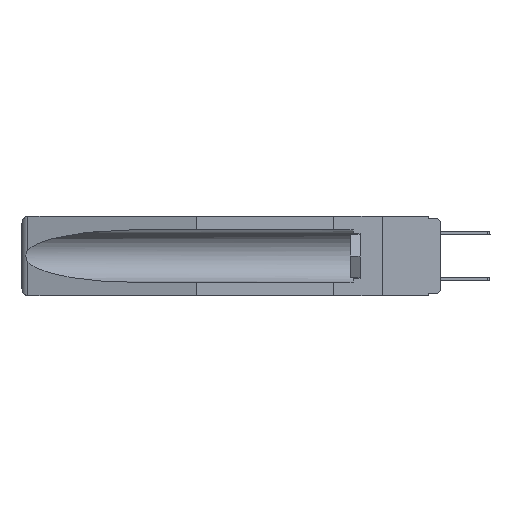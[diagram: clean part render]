
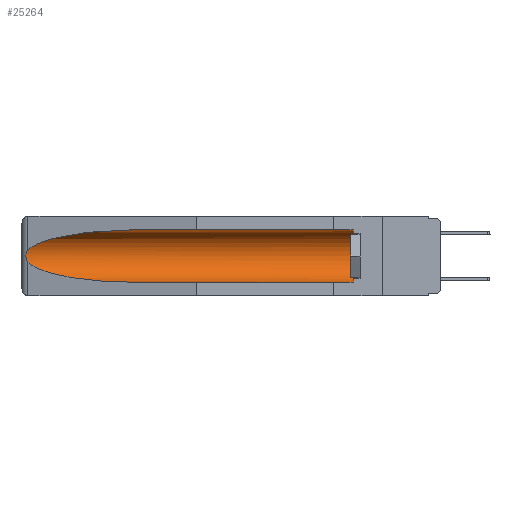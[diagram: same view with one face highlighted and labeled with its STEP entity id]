
A CAD part, left-side view. The second image highlights one B-rep face of the part: STEP entity #25264.
In plain terms, the highlighted cylindrical face has radius 2.857 mm (diameter 5.715 mm), a partial arc.
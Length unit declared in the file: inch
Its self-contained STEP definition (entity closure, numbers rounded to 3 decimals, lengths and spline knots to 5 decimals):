
#78 = CARTESIAN_POINT ( 'NONE',  ( 0.155, 0.126, -0.284 ) ) ;
#177 = DIRECTION ( 'NONE',  ( 0., 0., 1. ) ) ;
#429 = ORIENTED_EDGE ( 'NONE', *, *, #6052, .T. ) ;
#585 = EDGE_CURVE ( 'NONE', #12339, #21316, #16014, .T. ) ;
#729 = LINE ( 'NONE', #15188, #16115 ) ;
#1210 = CARTESIAN_POINT ( 'NONE',  ( 0.155, 1.07973, -0.059 ) ) ;
#1318 = CARTESIAN_POINT ( 'NONE',  ( 0.21114, 1.30732, -0.059 ) ) ;
#1515 = CARTESIAN_POINT ( 'NONE',  ( 0.25451, 1.48313, -0.24835 ) ) ;
#2762 = DIRECTION ( 'NONE',  ( 0., -1., 0. ) ) ;
#2861 = CARTESIAN_POINT ( 'NONE',  ( 0.155, 0.126, -0.059 ) ) ;
#3532 = CARTESIAN_POINT ( 'NONE',  ( 0.21114, 1.30732, -0.284 ) ) ;
#3777 = CARTESIAN_POINT ( 'NONE',  ( 0.26537, 1.52718, -0.14972 ) ) ;
#3855 = EDGE_CURVE ( 'NONE', #14499, #22951, #9195, .T. ) ;
#5232 =( BOUNDED_CURVE ( )  B_SPLINE_CURVE ( 3, ( #5443, #1318, #21371, #15358 ),
 .UNSPECIFIED., .F., .F. ) 
 B_SPLINE_CURVE_WITH_KNOTS ( ( 4, 4 ),
 ( 4.71239, 6.08839 ),
 .UNSPECIFIED. ) 
 CURVE ( )  GEOMETRIC_REPRESENTATION_ITEM ( )  RATIONAL_B_SPLINE_CURVE ( ( 1., 0.848, 0.848, 1. ) ) 
 REPRESENTATION_ITEM ( '' )  );
#5443 = CARTESIAN_POINT ( 'NONE',  ( 0.155, 1.07973, -0.059 ) ) ;
#5630 = CARTESIAN_POINT ( 'NONE',  ( 0.2673, 1.5327, -0.16383 ) ) ;
#5717 = CARTESIAN_POINT ( 'NONE',  ( 0.26655, 1.53094, -0.18657 ) ) ;
#5944 = CIRCLE ( 'NONE', #20447, 0.1125 ) ;
#6052 = EDGE_CURVE ( 'NONE', #9518, #14499, #5944, .T. ) ;
#6240 = CARTESIAN_POINT ( 'NONE',  ( 0.155, -0.30754, -0.1715 ) ) ;
#7721 = CARTESIAN_POINT ( 'NONE',  ( 0.2675, 1.53308, -0.16763 ) ) ;
#7921 = VECTOR ( 'NONE', #22058, 39.37008 ) ;
#9195 = LINE ( 'NONE', #10019, #7921 ) ;
#9518 = VERTEX_POINT ( 'NONE', #78 ) ;
#9766 = CARTESIAN_POINT ( 'NONE',  ( 0.26537, 1.52718, -0.14972 ) ) ;
#9856 = ORIENTED_EDGE ( 'NONE', *, *, #17966, .T. ) ;
#9872 = VERTEX_POINT ( 'NONE', #9766 ) ;
#9897 = ORIENTED_EDGE ( 'NONE', *, *, #3855, .T. ) ;
#10019 = CARTESIAN_POINT ( 'NONE',  ( 0.155, -0.30754, -0.059 ) ) ;
#12339 = VERTEX_POINT ( 'NONE', #22707 ) ;
#13170 = ORIENTED_EDGE ( 'NONE', *, *, #15056, .T. ) ;
#13279 = CYLINDRICAL_SURFACE ( 'NONE', #13897, 0.1125 ) ;
#13524 = EDGE_LOOP ( 'NONE', ( #13170, #9856, #25068, #18639, #429, #9897 ) ) ;
#13610 = FACE_OUTER_BOUND ( 'NONE', #13524, .T. ) ;
#13897 = AXIS2_PLACEMENT_3D ( 'NONE', #6240, #24117, #177 ) ;
#14499 = VERTEX_POINT ( 'NONE', #2861 ) ;
#15056 = EDGE_CURVE ( 'NONE', #22951, #9872, #5232, .T. ) ;
#15188 = CARTESIAN_POINT ( 'NONE',  ( 0.155, -0.30754, -0.284 ) ) ;
#15358 = CARTESIAN_POINT ( 'NONE',  ( 0.26537, 1.52718, -0.14972 ) ) ;
#15461 = CARTESIAN_POINT ( 'NONE',  ( 0.2675, 1.53308, -0.17534 ) ) ;
#15682 = B_SPLINE_CURVE_WITH_KNOTS ( 'NONE', 3,
 ( #3777, #17570, #15711, #5630, #7721, #15461, #21564, #5717, #21724, #17659 ),
 .UNSPECIFIED., .F., .F.,
 ( 4, 2, 2, 2, 4 ),
 ( 0., 0.00029, 0.00058, 0.00087, 0.00117 ),
 .UNSPECIFIED. ) ;
#15711 = CARTESIAN_POINT ( 'NONE',  ( 0.26654, 1.53092, -0.15636 ) ) ;
#16014 =( BOUNDED_CURVE ( )  B_SPLINE_CURVE ( 3, ( #21309, #1515, #3532, #23588 ),
 .UNSPECIFIED., .F., .T. ) 
 B_SPLINE_CURVE_WITH_KNOTS ( ( 4, 4 ),
 ( 0.1948, 1.5708 ),
 .UNSPECIFIED. ) 
 CURVE ( )  GEOMETRIC_REPRESENTATION_ITEM ( )  RATIONAL_B_SPLINE_CURVE ( ( 1., 0.848, 0.848, 1. ) ) 
 REPRESENTATION_ITEM ( '' )  );
#16115 = VECTOR ( 'NONE', #25255, 39.37008 ) ;
#16858 = EDGE_CURVE ( 'NONE', #9518, #21316, #729, .T. ) ;
#17570 = CARTESIAN_POINT ( 'NONE',  ( 0.26597, 1.52961, -0.15275 ) ) ;
#17659 = CARTESIAN_POINT ( 'NONE',  ( 0.26537, 1.52718, -0.19328 ) ) ;
#17966 = EDGE_CURVE ( 'NONE', #9872, #12339, #15682, .T. ) ;
#18639 = ORIENTED_EDGE ( 'NONE', *, *, #16858, .F. ) ;
#20447 = AXIS2_PLACEMENT_3D ( 'NONE', #24669, #2762, #24575 ) ;
#21309 = CARTESIAN_POINT ( 'NONE',  ( 0.26537, 1.52718, -0.19328 ) ) ;
#21316 = VERTEX_POINT ( 'NONE', #25926 ) ;
#21371 = CARTESIAN_POINT ( 'NONE',  ( 0.25451, 1.48313, -0.09465 ) ) ;
#21564 = CARTESIAN_POINT ( 'NONE',  ( 0.2673, 1.53269, -0.17917 ) ) ;
#21724 = CARTESIAN_POINT ( 'NONE',  ( 0.26597, 1.5296, -0.19026 ) ) ;
#22058 = DIRECTION ( 'NONE',  ( 0., 1., 0. ) ) ;
#22707 = CARTESIAN_POINT ( 'NONE',  ( 0.26537, 1.52718, -0.19328 ) ) ;
#22951 = VERTEX_POINT ( 'NONE', #1210 ) ;
#23588 = CARTESIAN_POINT ( 'NONE',  ( 0.155, 1.07973, -0.284 ) ) ;
#24117 = DIRECTION ( 'NONE',  ( 0., 1., 0. ) ) ;
#24575 = DIRECTION ( 'NONE',  ( 0., 0., 1. ) ) ;
#24669 = CARTESIAN_POINT ( 'NONE',  ( 0.155, 0.126, -0.1715 ) ) ;
#25068 = ORIENTED_EDGE ( 'NONE', *, *, #585, .T. ) ;
#25255 = DIRECTION ( 'NONE',  ( 0., 1., 0. ) ) ;
#25264 = ADVANCED_FACE ( 'NONE', ( #13610 ), #13279, .F. ) ;
#25926 = CARTESIAN_POINT ( 'NONE',  ( 0.155, 1.07973, -0.284 ) ) ;
